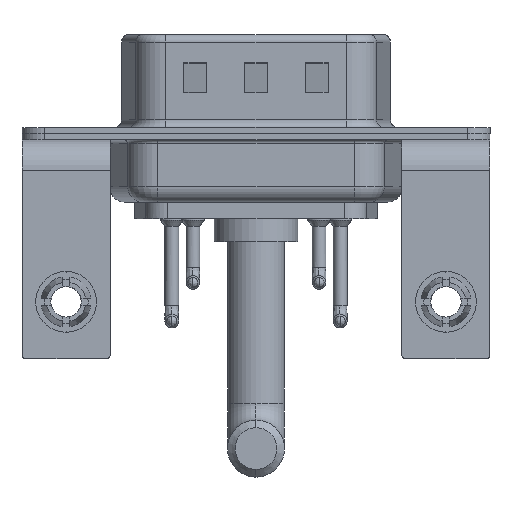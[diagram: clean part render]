
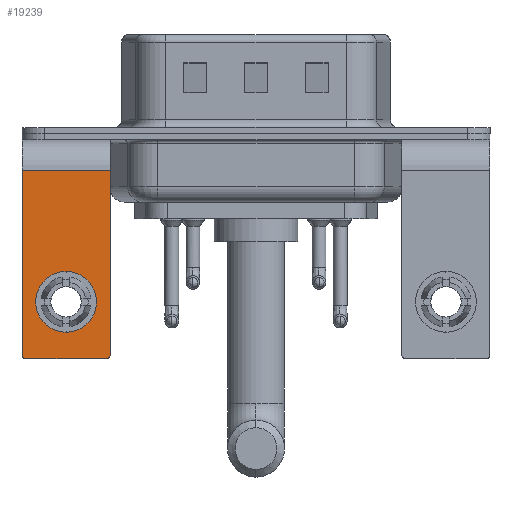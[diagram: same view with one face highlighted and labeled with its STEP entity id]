
A CAD part, front view. The second image highlights one B-rep face of the part: STEP entity #19239.
In plain terms, the highlighted planar face has unit normal (0, -1, 0).
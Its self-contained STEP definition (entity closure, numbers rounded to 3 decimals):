
#164 = LINE ( 'NONE', #6930, #17751 ) ;
#402 = CARTESIAN_POINT ( 'NONE',  ( 2.9, -6.25, -2.4 ) ) ;
#938 = ORIENTED_EDGE ( 'NONE', *, *, #19694, .F. ) ;
#967 = DIRECTION ( 'NONE',  ( 0., 1., 0. ) ) ;
#1007 = EDGE_CURVE ( 'NONE', #14991, #15603, #3856, .T. ) ;
#1282 = EDGE_CURVE ( 'NONE', #3025, #7919, #20511, .T. ) ;
#1413 = CARTESIAN_POINT ( 'NONE',  ( 2.9, -6.25, -2.4 ) ) ;
#1414 = AXIS2_PLACEMENT_3D ( 'NONE', #21593, #13176, #7762 ) ;
#1568 = EDGE_LOOP ( 'NONE', ( #19819, #19257 ) ) ;
#3025 = VERTEX_POINT ( 'NONE', #11472 ) ;
#3856 = CIRCLE ( 'NONE', #16265, 2. ) ;
#4627 = DIRECTION ( 'NONE',  ( -1., 0., 0. ) ) ;
#5528 = AXIS2_PLACEMENT_3D ( 'NONE', #11050, #967, #7739 ) ;
#6170 = VECTOR ( 'NONE', #4627, 1000. ) ;
#6930 = CARTESIAN_POINT ( 'NONE',  ( 2.9, -6.25, -14.8 ) ) ;
#7423 = EDGE_CURVE ( 'NONE', #10430, #8635, #10415, .T. ) ;
#7685 = DIRECTION ( 'NONE',  ( 0., -1., 0. ) ) ;
#7739 = DIRECTION ( 'NONE',  ( 0., 0., 1. ) ) ;
#7762 = DIRECTION ( 'NONE',  ( 0., 0., 1. ) ) ;
#7919 = VERTEX_POINT ( 'NONE', #11670 ) ;
#8635 = VERTEX_POINT ( 'NONE', #19713 ) ;
#8649 = DIRECTION ( 'NONE',  ( 0., 0., 1. ) ) ;
#8761 = DIRECTION ( 'NONE',  ( 0., 1., 0. ) ) ;
#9111 = EDGE_CURVE ( 'NONE', #15603, #14991, #19336, .T. ) ;
#9279 = EDGE_CURVE ( 'NONE', #8635, #17682, #21448, .T. ) ;
#9342 = DIRECTION ( 'NONE',  ( 0., 0., 1. ) ) ;
#10206 = DIRECTION ( 'NONE',  ( 0., 0., 1. ) ) ;
#10377 = CARTESIAN_POINT ( 'NONE',  ( 0., -6.25, -13.07 ) ) ;
#10415 = LINE ( 'NONE', #13746, #11123 ) ;
#10430 = VERTEX_POINT ( 'NONE', #14251 ) ;
#10692 = DIRECTION ( 'NONE',  ( -1., 0., 0. ) ) ;
#11050 = CARTESIAN_POINT ( 'NONE',  ( 0., -6.25, -11.07 ) ) ;
#11123 = VECTOR ( 'NONE', #19043, 1000. ) ;
#11472 = CARTESIAN_POINT ( 'NONE',  ( 2.65, -6.25, -14.8 ) ) ;
#11514 = EDGE_CURVE ( 'NONE', #11867, #10430, #17932, .T. ) ;
#11666 = EDGE_LOOP ( 'NONE', ( #15345, #18161, #938, #20844, #16429, #21001 ) ) ;
#11670 = CARTESIAN_POINT ( 'NONE',  ( 2.9, -6.25, -14.55 ) ) ;
#11867 = VERTEX_POINT ( 'NONE', #402 ) ;
#12083 = PLANE ( 'NONE',  #18793 ) ;
#12629 = AXIS2_PLACEMENT_3D ( 'NONE', #17762, #7685, #9342 ) ;
#13176 = DIRECTION ( 'NONE',  ( 0., -1., 0. ) ) ;
#13746 = CARTESIAN_POINT ( 'NONE',  ( -2.9, -6.25, -2.4 ) ) ;
#13846 = CARTESIAN_POINT ( 'NONE',  ( 0., -6.25, -9.07 ) ) ;
#14251 = CARTESIAN_POINT ( 'NONE',  ( -2.9, -6.25, -2.4 ) ) ;
#14492 = FACE_OUTER_BOUND ( 'NONE', #11666, .T. ) ;
#14631 = CARTESIAN_POINT ( 'NONE',  ( -2.65, -6.25, -14.8 ) ) ;
#14991 = VERTEX_POINT ( 'NONE', #13846 ) ;
#15345 = ORIENTED_EDGE ( 'NONE', *, *, #7423, .T. ) ;
#15530 = CARTESIAN_POINT ( 'NONE',  ( 2.9, -6.25, -2.4 ) ) ;
#15603 = VERTEX_POINT ( 'NONE', #10377 ) ;
#16265 = AXIS2_PLACEMENT_3D ( 'NONE', #17316, #18849, #10206 ) ;
#16429 = ORIENTED_EDGE ( 'NONE', *, *, #19766, .F. ) ;
#17316 = CARTESIAN_POINT ( 'NONE',  ( 0., -6.25, -11.07 ) ) ;
#17464 = DIRECTION ( 'NONE',  ( 0., 0., -1. ) ) ;
#17674 = LINE ( 'NONE', #20650, #18808 ) ;
#17682 = VERTEX_POINT ( 'NONE', #14631 ) ;
#17751 = VECTOR ( 'NONE', #10692, 1000. ) ;
#17762 = CARTESIAN_POINT ( 'NONE',  ( -2.65, -6.25, -14.55 ) ) ;
#17932 = LINE ( 'NONE', #1413, #6170 ) ;
#18161 = ORIENTED_EDGE ( 'NONE', *, *, #9279, .T. ) ;
#18793 = AXIS2_PLACEMENT_3D ( 'NONE', #15530, #8761, #8649 ) ;
#18808 = VECTOR ( 'NONE', #17464, 1000. ) ;
#18849 = DIRECTION ( 'NONE',  ( 0., 1., 0. ) ) ;
#19043 = DIRECTION ( 'NONE',  ( 0., 0., -1. ) ) ;
#19239 = ADVANCED_FACE ( 'NONE', ( #21226, #14492 ), #12083, .F. ) ;
#19257 = ORIENTED_EDGE ( 'NONE', *, *, #1007, .T. ) ;
#19336 = CIRCLE ( 'NONE', #5528, 2. ) ;
#19694 = EDGE_CURVE ( 'NONE', #3025, #17682, #164, .T. ) ;
#19713 = CARTESIAN_POINT ( 'NONE',  ( -2.9, -6.25, -14.55 ) ) ;
#19766 = EDGE_CURVE ( 'NONE', #11867, #7919, #17674, .T. ) ;
#19819 = ORIENTED_EDGE ( 'NONE', *, *, #9111, .T. ) ;
#20511 = CIRCLE ( 'NONE', #1414, 0.25 ) ;
#20650 = CARTESIAN_POINT ( 'NONE',  ( 2.9, -6.25, -2.4 ) ) ;
#20844 = ORIENTED_EDGE ( 'NONE', *, *, #1282, .T. ) ;
#21001 = ORIENTED_EDGE ( 'NONE', *, *, #11514, .T. ) ;
#21226 = FACE_BOUND ( 'NONE', #1568, .T. ) ;
#21448 = CIRCLE ( 'NONE', #12629, 0.25 ) ;
#21593 = CARTESIAN_POINT ( 'NONE',  ( 2.65, -6.25, -14.55 ) ) ;
